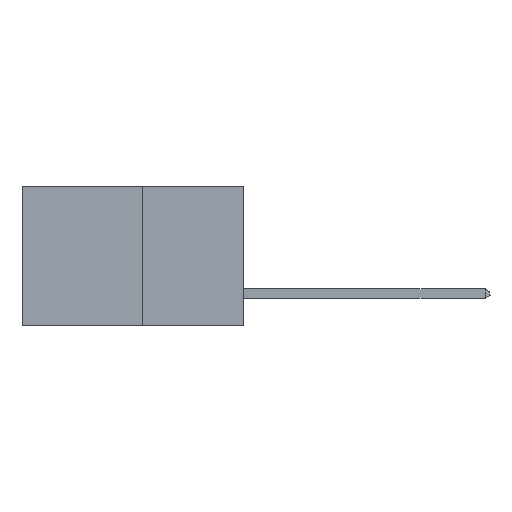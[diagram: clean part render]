
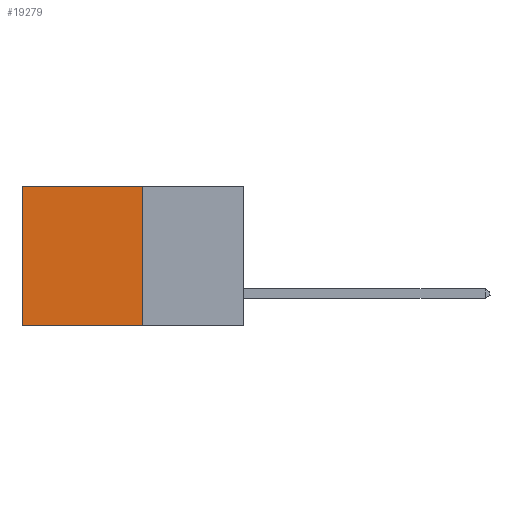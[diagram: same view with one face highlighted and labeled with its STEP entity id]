
A CAD part, left-side view. The second image highlights one B-rep face of the part: STEP entity #19279.
In plain terms, the highlighted planar face has unit normal (-1, 0, 0).
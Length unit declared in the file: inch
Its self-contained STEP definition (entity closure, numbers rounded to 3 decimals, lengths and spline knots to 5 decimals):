
#1485 = PLANE ( 'NONE',  #7776 ) ;
#2116 = VECTOR ( 'NONE', #13170, 39.37008 ) ;
#2686 = EDGE_CURVE ( 'NONE', #4843, #11265, #17984, .T. ) ;
#2752 = ORIENTED_EDGE ( 'NONE', *, *, #18469, .T. ) ;
#3124 = VECTOR ( 'NONE', #23500, 39.37008 ) ;
#3296 = FACE_OUTER_BOUND ( 'NONE', #21839, .T. ) ;
#3747 = CARTESIAN_POINT ( 'NONE',  ( 0.277, 0.59, -0.37 ) ) ;
#4843 = VERTEX_POINT ( 'NONE', #7703 ) ;
#5315 = CARTESIAN_POINT ( 'NONE',  ( 0.277, 0.27, -0.37 ) ) ;
#6938 = ORIENTED_EDGE ( 'NONE', *, *, #15065, .F. ) ;
#7239 = DIRECTION ( 'NONE',  ( 0., 0., -1. ) ) ;
#7703 = CARTESIAN_POINT ( 'NONE',  ( 0.277, 0.27, 0. ) ) ;
#7776 = AXIS2_PLACEMENT_3D ( 'NONE', #5315, #18300, #7239 ) ;
#8109 = LINE ( 'NONE', #14382, #17339 ) ;
#8232 = LINE ( 'NONE', #18233, #17475 ) ;
#8895 = DIRECTION ( 'NONE',  ( 0., 0., -1. ) ) ;
#11265 = VERTEX_POINT ( 'NONE', #12730 ) ;
#12697 = DIRECTION ( 'NONE',  ( 0., 1., 0. ) ) ;
#12730 = CARTESIAN_POINT ( 'NONE',  ( 0.277, 0.59, 0. ) ) ;
#13170 = DIRECTION ( 'NONE',  ( 0., 0., -1. ) ) ;
#14382 = CARTESIAN_POINT ( 'NONE',  ( 0.277, 0.27, -0.37 ) ) ;
#14796 = ORIENTED_EDGE ( 'NONE', *, *, #2686, .T. ) ;
#15065 = EDGE_CURVE ( 'NONE', #19706, #21595, #8232, .T. ) ;
#17037 = LINE ( 'NONE', #3747, #2116 ) ;
#17339 = VECTOR ( 'NONE', #8895, 39.37008 ) ;
#17475 = VECTOR ( 'NONE', #12697, 39.37008 ) ;
#17984 = LINE ( 'NONE', #22351, #3124 ) ;
#18233 = CARTESIAN_POINT ( 'NONE',  ( 0.277, 0.27, -0.37 ) ) ;
#18248 = EDGE_CURVE ( 'NONE', #4843, #19706, #8109, .T. ) ;
#18300 = DIRECTION ( 'NONE',  ( 1., 0., 0. ) ) ;
#18469 = EDGE_CURVE ( 'NONE', #11265, #21595, #17037, .T. ) ;
#19279 = ADVANCED_FACE ( 'NONE', ( #3296 ), #1485, .F. ) ;
#19424 = CARTESIAN_POINT ( 'NONE',  ( 0.277, 0.59, -0.37 ) ) ;
#19706 = VERTEX_POINT ( 'NONE', #23116 ) ;
#21595 = VERTEX_POINT ( 'NONE', #19424 ) ;
#21839 = EDGE_LOOP ( 'NONE', ( #2752, #6938, #23409, #14796 ) ) ;
#22351 = CARTESIAN_POINT ( 'NONE',  ( 0.277, 0.27, 0. ) ) ;
#23116 = CARTESIAN_POINT ( 'NONE',  ( 0.277, 0.27, -0.37 ) ) ;
#23409 = ORIENTED_EDGE ( 'NONE', *, *, #18248, .F. ) ;
#23500 = DIRECTION ( 'NONE',  ( 0., 1., 0. ) ) ;
